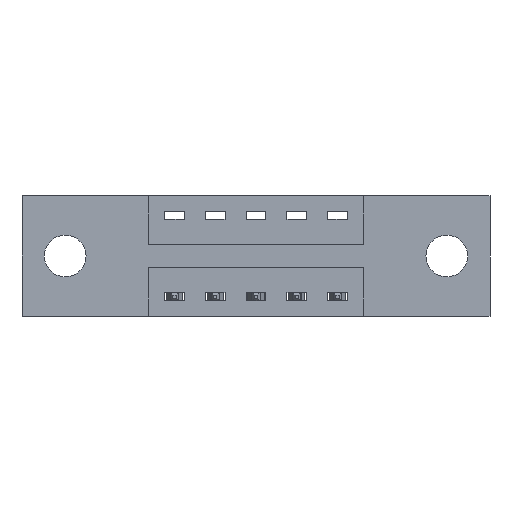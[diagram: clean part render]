
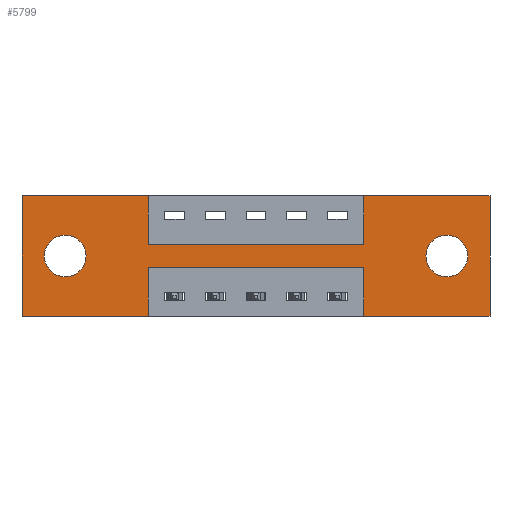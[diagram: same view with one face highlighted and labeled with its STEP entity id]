
A CAD part, front view. The second image highlights one B-rep face of the part: STEP entity #5799.
In plain terms, the highlighted planar face has unit normal (0, -1, 0).
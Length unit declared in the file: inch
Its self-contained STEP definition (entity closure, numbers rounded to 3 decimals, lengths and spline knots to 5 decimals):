
#89 = ORIENTED_EDGE ( 'NONE', *, *, #5924, .F. ) ;
#99 = DIRECTION ( 'NONE',  ( 0., 0., -1. ) ) ;
#221 = EDGE_CURVE ( 'NONE', #3862, #7187, #1671, .T. ) ;
#308 = VECTOR ( 'NONE', #6160, 39.37008 ) ;
#351 = VERTEX_POINT ( 'NONE', #607 ) ;
#375 = VERTEX_POINT ( 'NONE', #2527 ) ;
#441 = VERTEX_POINT ( 'NONE', #1235 ) ;
#496 = VERTEX_POINT ( 'NONE', #1361 ) ;
#577 = VECTOR ( 'NONE', #4306, 39.37008 ) ;
#607 = CARTESIAN_POINT ( 'NONE',  ( 0.1325, 0., -0.249 ) ) ;
#614 = CARTESIAN_POINT ( 'NONE',  ( 1.0475, 0., -0.37 ) ) ;
#629 = DIRECTION ( 'NONE',  ( 1., 0., 0. ) ) ;
#665 = EDGE_LOOP ( 'NONE', ( #3894, #2382 ) ) ;
#716 = LINE ( 'NONE', #3281, #7778 ) ;
#803 = CARTESIAN_POINT ( 'NONE',  ( 1.435, 0., 0. ) ) ;
#806 = CARTESIAN_POINT ( 'NONE',  ( 0., 0., -0.37 ) ) ;
#875 = EDGE_CURVE ( 'NONE', #4700, #2829, #7121, .T. ) ;
#930 = EDGE_CURVE ( 'NONE', #2829, #5680, #6734, .T. ) ;
#956 = VERTEX_POINT ( 'NONE', #4922 ) ;
#1096 = DIRECTION ( 'NONE',  ( 1., 0., 0. ) ) ;
#1235 = CARTESIAN_POINT ( 'NONE',  ( 0.1325, 0., -0.121 ) ) ;
#1317 = PLANE ( 'NONE',  #2577 ) ;
#1361 = CARTESIAN_POINT ( 'NONE',  ( 0.3875, 0., -0.15 ) ) ;
#1468 = EDGE_CURVE ( 'NONE', #956, #375, #1776, .T. ) ;
#1554 = ORIENTED_EDGE ( 'NONE', *, *, #6386, .F. ) ;
#1567 = ORIENTED_EDGE ( 'NONE', *, *, #7239, .F. ) ;
#1576 = EDGE_CURVE ( 'NONE', #7895, #6458, #6691, .T. ) ;
#1671 = LINE ( 'NONE', #7335, #3389 ) ;
#1680 = DIRECTION ( 'NONE',  ( 0., 1., 0. ) ) ;
#1729 = CARTESIAN_POINT ( 'NONE',  ( 0., 0., -0.37 ) ) ;
#1776 = LINE ( 'NONE', #1940, #6553 ) ;
#1804 = DIRECTION ( 'NONE',  ( 0., 0., 1. ) ) ;
#1809 = CIRCLE ( 'NONE', #3898, 0.064 ) ;
#1940 = CARTESIAN_POINT ( 'NONE',  ( 0.3875, 0., -0.22 ) ) ;
#2284 = DIRECTION ( 'NONE',  ( 0., 1., 0. ) ) ;
#2358 = DIRECTION ( 'NONE',  ( 0., 1., 0. ) ) ;
#2382 = ORIENTED_EDGE ( 'NONE', *, *, #1576, .T. ) ;
#2400 = EDGE_LOOP ( 'NONE', ( #2783, #7147 ) ) ;
#2527 = CARTESIAN_POINT ( 'NONE',  ( 0.3875, 0., -0.22 ) ) ;
#2531 = CARTESIAN_POINT ( 'NONE',  ( 0.3875, 0., 0. ) ) ;
#2577 = AXIS2_PLACEMENT_3D ( 'NONE', #6216, #6960, #7623 ) ;
#2604 = FACE_OUTER_BOUND ( 'NONE', #4746, .T. ) ;
#2650 = ORIENTED_EDGE ( 'NONE', *, *, #1468, .F. ) ;
#2696 = LINE ( 'NONE', #7062, #7378 ) ;
#2724 = VECTOR ( 'NONE', #8093, 39.37008 ) ;
#2783 = ORIENTED_EDGE ( 'NONE', *, *, #5291, .T. ) ;
#2829 = VERTEX_POINT ( 'NONE', #7477 ) ;
#2953 = ORIENTED_EDGE ( 'NONE', *, *, #3943, .F. ) ;
#2985 = DIRECTION ( 'NONE',  ( 0., 0., -1. ) ) ;
#3045 = ORIENTED_EDGE ( 'NONE', *, *, #6935, .F. ) ;
#3083 = CARTESIAN_POINT ( 'NONE',  ( 0.3875, 0., 0. ) ) ;
#3109 = CARTESIAN_POINT ( 'NONE',  ( 0., 0., 0. ) ) ;
#3130 = EDGE_CURVE ( 'NONE', #5680, #956, #2696, .T. ) ;
#3213 = CARTESIAN_POINT ( 'NONE',  ( 1.0475, 0., 0. ) ) ;
#3281 = CARTESIAN_POINT ( 'NONE',  ( 0.3875, 0., -0.15 ) ) ;
#3388 = AXIS2_PLACEMENT_3D ( 'NONE', #5408, #2284, #6056 ) ;
#3389 = VECTOR ( 'NONE', #1804, 39.37008 ) ;
#3463 = EDGE_CURVE ( 'NONE', #6458, #7895, #1809, .T. ) ;
#3500 = CARTESIAN_POINT ( 'NONE',  ( 1.3025, 0., -0.185 ) ) ;
#3689 = VERTEX_POINT ( 'NONE', #7842 ) ;
#3703 = DIRECTION ( 'NONE',  ( -1., 0., 0. ) ) ;
#3834 = VERTEX_POINT ( 'NONE', #4335 ) ;
#3862 = VERTEX_POINT ( 'NONE', #806 ) ;
#3882 = ORIENTED_EDGE ( 'NONE', *, *, #221, .F. ) ;
#3883 = CARTESIAN_POINT ( 'NONE',  ( 0., 0., 0. ) ) ;
#3894 = ORIENTED_EDGE ( 'NONE', *, *, #3463, .T. ) ;
#3898 = AXIS2_PLACEMENT_3D ( 'NONE', #6025, #1680, #6678 ) ;
#3943 = EDGE_CURVE ( 'NONE', #3689, #4700, #7988, .T. ) ;
#4091 = DIRECTION ( 'NONE',  ( 0., 0., -1. ) ) ;
#4093 = ORIENTED_EDGE ( 'NONE', *, *, #875, .F. ) ;
#4264 = AXIS2_PLACEMENT_3D ( 'NONE', #4678, #2358, #7325 ) ;
#4306 = DIRECTION ( 'NONE',  ( 0., 0., -1. ) ) ;
#4335 = CARTESIAN_POINT ( 'NONE',  ( 1.0475, 0., -0.15 ) ) ;
#4549 = DIRECTION ( 'NONE',  ( 0., 0., 1. ) ) ;
#4606 = CARTESIAN_POINT ( 'NONE',  ( 0., 0., -0.37 ) ) ;
#4625 = VECTOR ( 'NONE', #7838, 39.37008 ) ;
#4678 = CARTESIAN_POINT ( 'NONE',  ( 0.1325, 0., -0.185 ) ) ;
#4700 = VERTEX_POINT ( 'NONE', #7616 ) ;
#4746 = EDGE_LOOP ( 'NONE', ( #1554, #2650, #6496, #5044, #4093, #2953, #3045, #5660, #7837, #89, #3882, #1567 ) ) ;
#4853 = AXIS2_PLACEMENT_3D ( 'NONE', #3500, #6027, #4091 ) ;
#4901 = CIRCLE ( 'NONE', #4264, 0.064 ) ;
#4922 = CARTESIAN_POINT ( 'NONE',  ( 1.0475, 0., -0.22 ) ) ;
#5044 = ORIENTED_EDGE ( 'NONE', *, *, #930, .F. ) ;
#5107 = FACE_BOUND ( 'NONE', #2400, .T. ) ;
#5175 = LINE ( 'NONE', #3213, #7264 ) ;
#5275 = LINE ( 'NONE', #4606, #4625 ) ;
#5291 = EDGE_CURVE ( 'NONE', #441, #351, #6875, .T. ) ;
#5358 = LINE ( 'NONE', #6834, #308 ) ;
#5399 = EDGE_CURVE ( 'NONE', #351, #441, #4901, .T. ) ;
#5408 = CARTESIAN_POINT ( 'NONE',  ( 0.1325, 0., -0.185 ) ) ;
#5660 = ORIENTED_EDGE ( 'NONE', *, *, #6521, .F. ) ;
#5680 = VERTEX_POINT ( 'NONE', #614 ) ;
#5760 = CARTESIAN_POINT ( 'NONE',  ( 1.3025, 0., -0.249 ) ) ;
#5799 = ADVANCED_FACE ( 'NONE', ( #6254, #5107, #2604 ), #1317, .T. ) ;
#5924 = EDGE_CURVE ( 'NONE', #7187, #7097, #5358, .T. ) ;
#6025 = CARTESIAN_POINT ( 'NONE',  ( 1.3025, 0., -0.185 ) ) ;
#6027 = DIRECTION ( 'NONE',  ( 0., 1., 0. ) ) ;
#6056 = DIRECTION ( 'NONE',  ( 0., 0., 1. ) ) ;
#6160 = DIRECTION ( 'NONE',  ( 1., 0., 0. ) ) ;
#6216 = CARTESIAN_POINT ( 'NONE',  ( 0., 0., -0.37 ) ) ;
#6254 = FACE_BOUND ( 'NONE', #665, .T. ) ;
#6386 = EDGE_CURVE ( 'NONE', #375, #7360, #6656, .T. ) ;
#6458 = VERTEX_POINT ( 'NONE', #6994 ) ;
#6496 = ORIENTED_EDGE ( 'NONE', *, *, #3130, .F. ) ;
#6521 = EDGE_CURVE ( 'NONE', #496, #3834, #716, .T. ) ;
#6553 = VECTOR ( 'NONE', #3703, 39.37008 ) ;
#6656 = LINE ( 'NONE', #7869, #7552 ) ;
#6678 = DIRECTION ( 'NONE',  ( 0., 0., -1. ) ) ;
#6691 = CIRCLE ( 'NONE', #4853, 0.064 ) ;
#6734 = LINE ( 'NONE', #1729, #2724 ) ;
#6834 = CARTESIAN_POINT ( 'NONE',  ( 0., 0., 0. ) ) ;
#6875 = CIRCLE ( 'NONE', #3388, 0.064 ) ;
#6935 = EDGE_CURVE ( 'NONE', #3834, #3689, #5175, .T. ) ;
#6960 = DIRECTION ( 'NONE',  ( 0., -1., 0. ) ) ;
#6994 = CARTESIAN_POINT ( 'NONE',  ( 1.3025, 0., -0.121 ) ) ;
#7013 = VECTOR ( 'NONE', #99, 39.37008 ) ;
#7062 = CARTESIAN_POINT ( 'NONE',  ( 1.0475, 0., -0.37 ) ) ;
#7097 = VERTEX_POINT ( 'NONE', #2531 ) ;
#7121 = LINE ( 'NONE', #803, #7013 ) ;
#7147 = ORIENTED_EDGE ( 'NONE', *, *, #5399, .T. ) ;
#7150 = EDGE_CURVE ( 'NONE', #7097, #496, #7999, .T. ) ;
#7187 = VERTEX_POINT ( 'NONE', #3883 ) ;
#7239 = EDGE_CURVE ( 'NONE', #7360, #3862, #5275, .T. ) ;
#7264 = VECTOR ( 'NONE', #4549, 39.37008 ) ;
#7325 = DIRECTION ( 'NONE',  ( 0., 0., 1. ) ) ;
#7329 = CARTESIAN_POINT ( 'NONE',  ( 0.3875, 0., -0.37 ) ) ;
#7335 = CARTESIAN_POINT ( 'NONE',  ( 0., 0., 0. ) ) ;
#7360 = VERTEX_POINT ( 'NONE', #7329 ) ;
#7378 = VECTOR ( 'NONE', #7597, 39.37008 ) ;
#7477 = CARTESIAN_POINT ( 'NONE',  ( 1.435, 0., -0.37 ) ) ;
#7552 = VECTOR ( 'NONE', #2985, 39.37008 ) ;
#7597 = DIRECTION ( 'NONE',  ( 0., 0., 1. ) ) ;
#7616 = CARTESIAN_POINT ( 'NONE',  ( 1.435, 0., 0. ) ) ;
#7623 = DIRECTION ( 'NONE',  ( 0., 0., -1. ) ) ;
#7778 = VECTOR ( 'NONE', #629, 39.37008 ) ;
#7837 = ORIENTED_EDGE ( 'NONE', *, *, #7150, .F. ) ;
#7838 = DIRECTION ( 'NONE',  ( -1., 0., 0. ) ) ;
#7842 = CARTESIAN_POINT ( 'NONE',  ( 1.0475, 0., 0. ) ) ;
#7869 = CARTESIAN_POINT ( 'NONE',  ( 0.3875, 0., -0.37 ) ) ;
#7895 = VERTEX_POINT ( 'NONE', #5760 ) ;
#7988 = LINE ( 'NONE', #3109, #8076 ) ;
#7999 = LINE ( 'NONE', #3083, #577 ) ;
#8076 = VECTOR ( 'NONE', #1096, 39.37008 ) ;
#8093 = DIRECTION ( 'NONE',  ( -1., 0., 0. ) ) ;
